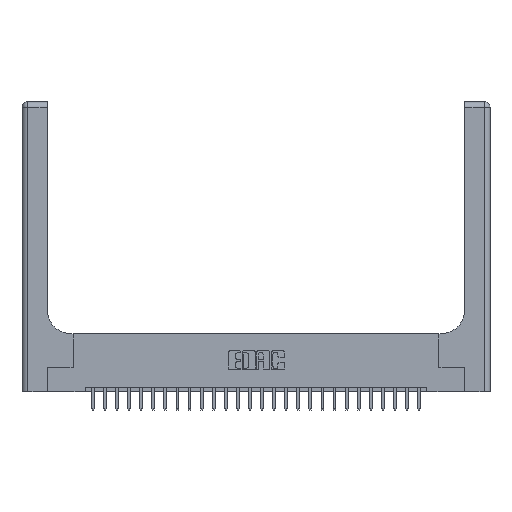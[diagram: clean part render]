
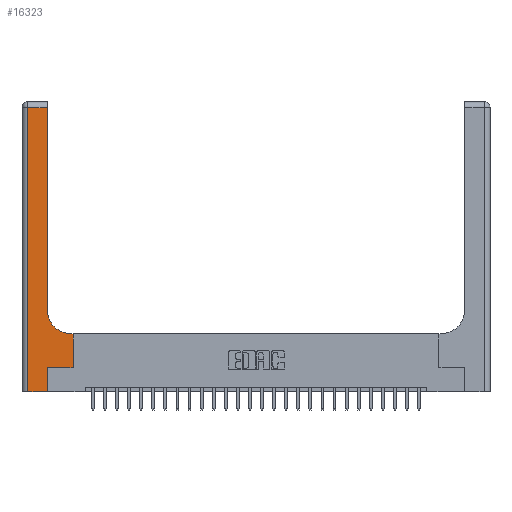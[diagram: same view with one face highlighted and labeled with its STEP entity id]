
A CAD part, top view. The second image highlights one B-rep face of the part: STEP entity #16323.
In plain terms, the highlighted planar face has unit normal (0, 0, 1).
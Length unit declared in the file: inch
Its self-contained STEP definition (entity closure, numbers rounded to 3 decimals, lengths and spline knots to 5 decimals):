
#96 = VECTOR ( 'NONE', #9677, 39.37008 ) ;
#266 = EDGE_CURVE ( 'NONE', #6999, #3275, #14136, .T. ) ;
#785 = ORIENTED_EDGE ( 'NONE', *, *, #266, .T. ) ;
#1164 = CARTESIAN_POINT ( 'NONE',  ( 0.06, 2.94, 0.37 ) ) ;
#1199 = VERTEX_POINT ( 'NONE', #1238 ) ;
#1238 = CARTESIAN_POINT ( 'NONE',  ( 0.06, 0., 0.37 ) ) ;
#1296 = DIRECTION ( 'NONE',  ( -1., 0., 0. ) ) ;
#2508 = DIRECTION ( 'NONE',  ( 0., 0., -1. ) ) ;
#2620 = CARTESIAN_POINT ( 'NONE',  ( 0., 0., 0.37 ) ) ;
#2762 = LINE ( 'NONE', #14617, #10174 ) ;
#2918 = VERTEX_POINT ( 'NONE', #20338 ) ;
#3275 = VERTEX_POINT ( 'NONE', #21633 ) ;
#3305 = VERTEX_POINT ( 'NONE', #23608 ) ;
#3416 = LINE ( 'NONE', #2620, #22181 ) ;
#3728 = LINE ( 'NONE', #5846, #14412 ) ;
#4424 = CARTESIAN_POINT ( 'NONE',  ( 0.265, 0.25, 0.37 ) ) ;
#5266 = CIRCLE ( 'NONE', #15713, 0.25 ) ;
#5846 = CARTESIAN_POINT ( 'NONE',  ( 0.06, 3., 0.37 ) ) ;
#5882 = LINE ( 'NONE', #23755, #96 ) ;
#6169 = EDGE_LOOP ( 'NONE', ( #12570, #19928, #15458, #21828, #20575, #17689, #785, #6865, #19337 ) ) ;
#6462 = EDGE_CURVE ( 'NONE', #2918, #3305, #20356, .T. ) ;
#6502 = EDGE_CURVE ( 'NONE', #13751, #6999, #5882, .T. ) ;
#6750 = DIRECTION ( 'NONE',  ( 0., 1., 0. ) ) ;
#6865 = ORIENTED_EDGE ( 'NONE', *, *, #22411, .T. ) ;
#6947 = VECTOR ( 'NONE', #6750, 39.37008 ) ;
#6999 = VERTEX_POINT ( 'NONE', #11124 ) ;
#8231 = FACE_OUTER_BOUND ( 'NONE', #6169, .T. ) ;
#8764 = CARTESIAN_POINT ( 'NONE',  ( 0.51, 0.6, 0.37 ) ) ;
#8863 = CARTESIAN_POINT ( 'NONE',  ( 0.265, 0., 0.37 ) ) ;
#9116 = DIRECTION ( 'NONE',  ( -1., 0., 0. ) ) ;
#9138 = PLANE ( 'NONE',  #11937 ) ;
#9318 = DIRECTION ( 'NONE',  ( 0., 0., -1. ) ) ;
#9677 = DIRECTION ( 'NONE',  ( 1., 0., 0. ) ) ;
#9825 = VERTEX_POINT ( 'NONE', #8764 ) ;
#10174 = VECTOR ( 'NONE', #9116, 39.37008 ) ;
#10553 = DIRECTION ( 'NONE',  ( 1., 0., 0. ) ) ;
#10742 = VECTOR ( 'NONE', #23422, 39.37008 ) ;
#11124 = CARTESIAN_POINT ( 'NONE',  ( 0.528, 0.25, 0.37 ) ) ;
#11663 = EDGE_CURVE ( 'NONE', #13133, #13751, #12537, .T. ) ;
#11937 = AXIS2_PLACEMENT_3D ( 'NONE', #15060, #9318, #15234 ) ;
#12444 = VERTEX_POINT ( 'NONE', #1164 ) ;
#12537 = LINE ( 'NONE', #8863, #6947 ) ;
#12570 = ORIENTED_EDGE ( 'NONE', *, *, #6462, .T. ) ;
#12679 = EDGE_CURVE ( 'NONE', #3305, #12444, #13030, .T. ) ;
#13030 = LINE ( 'NONE', #14722, #21967 ) ;
#13133 = VERTEX_POINT ( 'NONE', #22361 ) ;
#13751 = VERTEX_POINT ( 'NONE', #4424 ) ;
#13828 = EDGE_CURVE ( 'NONE', #1199, #13133, #3416, .T. ) ;
#14136 = LINE ( 'NONE', #15508, #10742 ) ;
#14412 = VECTOR ( 'NONE', #21790, 39.37008 ) ;
#14414 = EDGE_CURVE ( 'NONE', #9825, #2918, #5266, .T. ) ;
#14617 = CARTESIAN_POINT ( 'NONE',  ( 0.26, 0.6, 0.37 ) ) ;
#14722 = CARTESIAN_POINT ( 'NONE',  ( 0., 2.94, 0.37 ) ) ;
#15060 = CARTESIAN_POINT ( 'NONE',  ( 0., 3., 0.37 ) ) ;
#15234 = DIRECTION ( 'NONE',  ( -1., 0., 0. ) ) ;
#15458 = ORIENTED_EDGE ( 'NONE', *, *, #23956, .T. ) ;
#15508 = CARTESIAN_POINT ( 'NONE',  ( 0.528, 0.25, 0.37 ) ) ;
#15713 = AXIS2_PLACEMENT_3D ( 'NONE', #20402, #2508, #18144 ) ;
#15835 = DIRECTION ( 'NONE',  ( 0., 1., 0. ) ) ;
#16323 = ADVANCED_FACE ( 'NONE', ( #8231 ), #9138, .F. ) ;
#16353 = VECTOR ( 'NONE', #15835, 39.37008 ) ;
#17689 = ORIENTED_EDGE ( 'NONE', *, *, #6502, .T. ) ;
#18144 = DIRECTION ( 'NONE',  ( 1., 0., 0. ) ) ;
#19337 = ORIENTED_EDGE ( 'NONE', *, *, #14414, .T. ) ;
#19928 = ORIENTED_EDGE ( 'NONE', *, *, #12679, .T. ) ;
#20338 = CARTESIAN_POINT ( 'NONE',  ( 0.26, 0.85, 0.37 ) ) ;
#20356 = LINE ( 'NONE', #23673, #16353 ) ;
#20402 = CARTESIAN_POINT ( 'NONE',  ( 0.51, 0.85, 0.37 ) ) ;
#20575 = ORIENTED_EDGE ( 'NONE', *, *, #11663, .T. ) ;
#21633 = CARTESIAN_POINT ( 'NONE',  ( 0.528, 0.6, 0.37 ) ) ;
#21790 = DIRECTION ( 'NONE',  ( 0., -1., 0. ) ) ;
#21828 = ORIENTED_EDGE ( 'NONE', *, *, #13828, .T. ) ;
#21967 = VECTOR ( 'NONE', #1296, 39.37008 ) ;
#22181 = VECTOR ( 'NONE', #10553, 39.37008 ) ;
#22361 = CARTESIAN_POINT ( 'NONE',  ( 0.265, 0., 0.37 ) ) ;
#22411 = EDGE_CURVE ( 'NONE', #3275, #9825, #2762, .T. ) ;
#23422 = DIRECTION ( 'NONE',  ( 0., 1., 0. ) ) ;
#23608 = CARTESIAN_POINT ( 'NONE',  ( 0.26, 2.94, 0.37 ) ) ;
#23673 = CARTESIAN_POINT ( 'NONE',  ( 0.26, 3., 0.37 ) ) ;
#23755 = CARTESIAN_POINT ( 'NONE',  ( 0.265, 0.25, 0.37 ) ) ;
#23956 = EDGE_CURVE ( 'NONE', #12444, #1199, #3728, .T. ) ;
